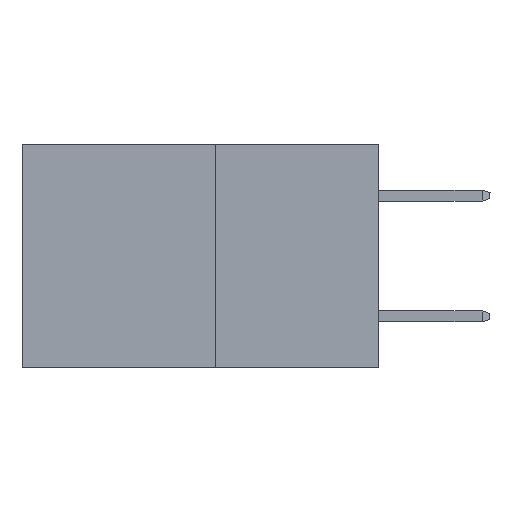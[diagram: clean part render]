
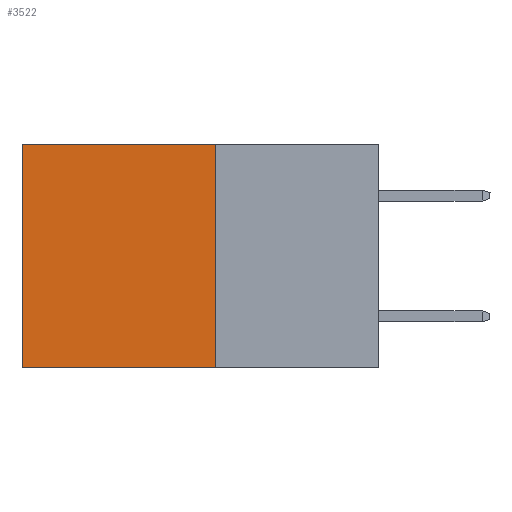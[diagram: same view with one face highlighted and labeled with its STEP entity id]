
A CAD part, left-side view. The second image highlights one B-rep face of the part: STEP entity #3522.
In plain terms, the highlighted planar face has unit normal (-1, 0, 0).
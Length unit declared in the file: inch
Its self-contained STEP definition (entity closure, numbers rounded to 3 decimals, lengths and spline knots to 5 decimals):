
#322 = EDGE_CURVE ( 'NONE', #6063, #2276, #6882, .T. ) ;
#574 = CARTESIAN_POINT ( 'NONE',  ( 0.277, 0.59, -0.37 ) ) ;
#600 = ORIENTED_EDGE ( 'NONE', *, *, #7835, .F. ) ;
#1278 = VERTEX_POINT ( 'NONE', #7803 ) ;
#1379 = VECTOR ( 'NONE', #5675, 39.37008 ) ;
#1798 = EDGE_CURVE ( 'NONE', #2276, #3357, #7608, .T. ) ;
#2123 = LINE ( 'NONE', #7153, #7356 ) ;
#2189 = CARTESIAN_POINT ( 'NONE',  ( 0.277, 0.59, 0. ) ) ;
#2276 = VERTEX_POINT ( 'NONE', #2189 ) ;
#2931 = CARTESIAN_POINT ( 'NONE',  ( 0.277, 0.59, -0.37 ) ) ;
#3245 = DIRECTION ( 'NONE',  ( 0., 0., -1. ) ) ;
#3357 = VERTEX_POINT ( 'NONE', #2931 ) ;
#3358 = CARTESIAN_POINT ( 'NONE',  ( 0.277, 0.27, -0.37 ) ) ;
#3409 = CARTESIAN_POINT ( 'NONE',  ( 0.277, 0.27, -0.37 ) ) ;
#3429 = DIRECTION ( 'NONE',  ( 1., 0., 0. ) ) ;
#3522 = ADVANCED_FACE ( 'NONE', ( #5724 ), #3757, .F. ) ;
#3757 = PLANE ( 'NONE',  #7756 ) ;
#3942 = EDGE_CURVE ( 'NONE', #6063, #1278, #2123, .T. ) ;
#4141 = VECTOR ( 'NONE', #8692, 39.37008 ) ;
#4784 = ORIENTED_EDGE ( 'NONE', *, *, #3942, .F. ) ;
#5415 = LINE ( 'NONE', #3358, #8904 ) ;
#5675 = DIRECTION ( 'NONE',  ( 0., 1., 0. ) ) ;
#5718 = CARTESIAN_POINT ( 'NONE',  ( 0.277, 0.27, 0. ) ) ;
#5724 = FACE_OUTER_BOUND ( 'NONE', #7570, .T. ) ;
#6063 = VERTEX_POINT ( 'NONE', #8442 ) ;
#6819 = DIRECTION ( 'NONE',  ( 0., 1., 0. ) ) ;
#6882 = LINE ( 'NONE', #5718, #1379 ) ;
#7018 = DIRECTION ( 'NONE',  ( 0., 0., -1. ) ) ;
#7153 = CARTESIAN_POINT ( 'NONE',  ( 0.277, 0.27, -0.37 ) ) ;
#7356 = VECTOR ( 'NONE', #7018, 39.37008 ) ;
#7570 = EDGE_LOOP ( 'NONE', ( #8389, #600, #4784, #7968 ) ) ;
#7608 = LINE ( 'NONE', #574, #4141 ) ;
#7756 = AXIS2_PLACEMENT_3D ( 'NONE', #3409, #3429, #3245 ) ;
#7803 = CARTESIAN_POINT ( 'NONE',  ( 0.277, 0.27, -0.37 ) ) ;
#7835 = EDGE_CURVE ( 'NONE', #1278, #3357, #5415, .T. ) ;
#7968 = ORIENTED_EDGE ( 'NONE', *, *, #322, .T. ) ;
#8389 = ORIENTED_EDGE ( 'NONE', *, *, #1798, .T. ) ;
#8442 = CARTESIAN_POINT ( 'NONE',  ( 0.277, 0.27, 0. ) ) ;
#8692 = DIRECTION ( 'NONE',  ( 0., 0., -1. ) ) ;
#8904 = VECTOR ( 'NONE', #6819, 39.37008 ) ;
